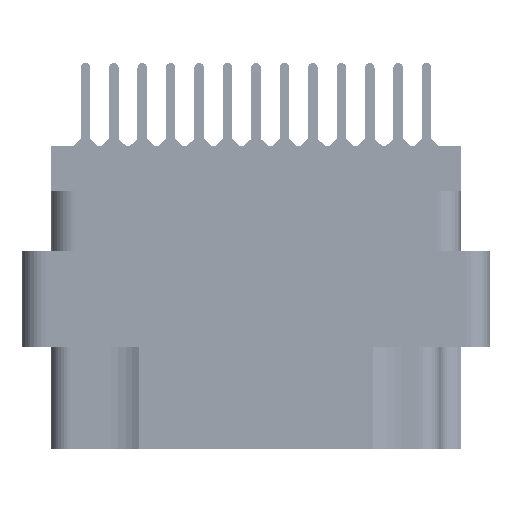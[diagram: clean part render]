
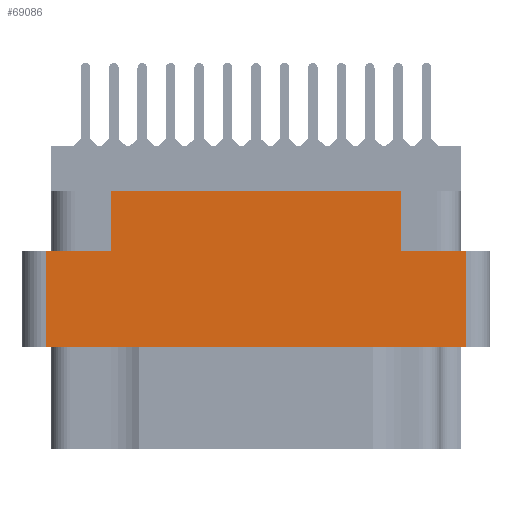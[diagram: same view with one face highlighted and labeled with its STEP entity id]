
A CAD part, left-side view. The second image highlights one B-rep face of the part: STEP entity #69086.
In plain terms, the highlighted planar face has unit normal (-1, 0, 0).
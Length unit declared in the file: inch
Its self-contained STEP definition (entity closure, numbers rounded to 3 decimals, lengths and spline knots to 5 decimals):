
#2115 = VERTEX_POINT ( 'NONE', #59527 ) ;
#8114 = ORIENTED_EDGE ( 'NONE', *, *, #72911, .F. ) ;
#8891 = ORIENTED_EDGE ( 'NONE', *, *, #37141, .T. ) ;
#9425 = VECTOR ( 'NONE', #20705, 39.37008 ) ;
#10020 = VECTOR ( 'NONE', #55788, 39.37008 ) ;
#10069 = DIRECTION ( 'NONE',  ( 0., 0., 1. ) ) ;
#10128 = CARTESIAN_POINT ( 'NONE',  ( -1.359, 0., -0.277 ) ) ;
#10649 = ORIENTED_EDGE ( 'NONE', *, *, #53684, .F. ) ;
#11189 = DIRECTION ( 'NONE',  ( -1., 0., 0. ) ) ;
#11497 = FACE_OUTER_BOUND ( 'NONE', #63966, .T. ) ;
#12118 = CARTESIAN_POINT ( 'NONE',  ( -1.359, -0.3825, -0.117 ) ) ;
#13114 = CARTESIAN_POINT ( 'NONE',  ( -1.359, 0.3825, -0.117 ) ) ;
#13892 = DIRECTION ( 'NONE',  ( 0., -1., 0. ) ) ;
#13907 = VERTEX_POINT ( 'NONE', #70611 ) ;
#17007 = EDGE_CURVE ( 'NONE', #26214, #62178, #38841, .T. ) ;
#17189 = VERTEX_POINT ( 'NONE', #28455 ) ;
#18447 = DIRECTION ( 'NONE',  ( 0., 0., 1. ) ) ;
#20012 = CARTESIAN_POINT ( 'NONE',  ( -1.359, 0.555, -0.798 ) ) ;
#20705 = DIRECTION ( 'NONE',  ( 0., 0., 1. ) ) ;
#21199 = DIRECTION ( 'NONE',  ( 0., -1., 0. ) ) ;
#21904 = CARTESIAN_POINT ( 'NONE',  ( -1.359, -0.555, -0.798 ) ) ;
#22113 = CARTESIAN_POINT ( 'NONE',  ( -1.359, 0.3825, -0.277 ) ) ;
#22502 = CARTESIAN_POINT ( 'NONE',  ( -1.359, -0.617, -0.798 ) ) ;
#25676 = CARTESIAN_POINT ( 'NONE',  ( -1.359, -0.555, -0.277 ) ) ;
#25785 = EDGE_CURVE ( 'NONE', #2115, #62178, #66826, .T. ) ;
#26214 = VERTEX_POINT ( 'NONE', #46643 ) ;
#26564 = VERTEX_POINT ( 'NONE', #67850 ) ;
#28455 = CARTESIAN_POINT ( 'NONE',  ( -1.359, 0.555, -0.277 ) ) ;
#29188 = LINE ( 'NONE', #44236, #9425 ) ;
#30741 = LINE ( 'NONE', #49799, #10020 ) ;
#30987 = CARTESIAN_POINT ( 'NONE',  ( -1.359, 0., -0.277 ) ) ;
#33061 = AXIS2_PLACEMENT_3D ( 'NONE', #22502, #11189, #18447 ) ;
#34282 = CARTESIAN_POINT ( 'NONE',  ( -1.359, 0., -0.529 ) ) ;
#34528 = DIRECTION ( 'NONE',  ( 0., 1., 0. ) ) ;
#35533 = EDGE_CURVE ( 'NONE', #17189, #13907, #43742, .T. ) ;
#37141 = EDGE_CURVE ( 'NONE', #2115, #40051, #29188, .T. ) ;
#38841 = LINE ( 'NONE', #21904, #63868 ) ;
#39416 = ORIENTED_EDGE ( 'NONE', *, *, #43409, .F. ) ;
#40051 = VERTEX_POINT ( 'NONE', #12118 ) ;
#40675 = ORIENTED_EDGE ( 'NONE', *, *, #17007, .T. ) ;
#42794 = ORIENTED_EDGE ( 'NONE', *, *, #25785, .F. ) ;
#43154 = VECTOR ( 'NONE', #60300, 39.37008 ) ;
#43409 = EDGE_CURVE ( 'NONE', #13907, #48974, #57511, .T. ) ;
#43742 = LINE ( 'NONE', #10128, #59783 ) ;
#44236 = CARTESIAN_POINT ( 'NONE',  ( -1.359, -0.3825, -0.277 ) ) ;
#44693 = ORIENTED_EDGE ( 'NONE', *, *, #35533, .F. ) ;
#46385 = LINE ( 'NONE', #34282, #54379 ) ;
#46643 = CARTESIAN_POINT ( 'NONE',  ( -1.359, -0.555, -0.529 ) ) ;
#48974 = VERTEX_POINT ( 'NONE', #13114 ) ;
#49799 = CARTESIAN_POINT ( 'NONE',  ( -1.359, 0.617, -0.117 ) ) ;
#51576 = VECTOR ( 'NONE', #13892, 39.37008 ) ;
#53684 = EDGE_CURVE ( 'NONE', #26214, #26564, #46385, .T. ) ;
#54379 = VECTOR ( 'NONE', #34528, 39.37008 ) ;
#55788 = DIRECTION ( 'NONE',  ( 0., -1., 0. ) ) ;
#56762 = PLANE ( 'NONE',  #33061 ) ;
#57511 = LINE ( 'NONE', #22113, #64702 ) ;
#57531 = EDGE_CURVE ( 'NONE', #17189, #26564, #67301, .T. ) ;
#58658 = ORIENTED_EDGE ( 'NONE', *, *, #57531, .T. ) ;
#59527 = CARTESIAN_POINT ( 'NONE',  ( -1.359, -0.3825, -0.277 ) ) ;
#59783 = VECTOR ( 'NONE', #21199, 39.37008 ) ;
#60300 = DIRECTION ( 'NONE',  ( 0., 0., -1. ) ) ;
#62178 = VERTEX_POINT ( 'NONE', #25676 ) ;
#63868 = VECTOR ( 'NONE', #68208, 39.37008 ) ;
#63966 = EDGE_LOOP ( 'NONE', ( #44693, #58658, #10649, #40675, #42794, #8891, #8114, #39416 ) ) ;
#64702 = VECTOR ( 'NONE', #10069, 39.37008 ) ;
#66826 = LINE ( 'NONE', #30987, #51576 ) ;
#67301 = LINE ( 'NONE', #20012, #43154 ) ;
#67850 = CARTESIAN_POINT ( 'NONE',  ( -1.359, 0.555, -0.529 ) ) ;
#68208 = DIRECTION ( 'NONE',  ( 0., 0., 1. ) ) ;
#69086 = ADVANCED_FACE ( 'NONE', ( #11497 ), #56762, .T. ) ;
#70611 = CARTESIAN_POINT ( 'NONE',  ( -1.359, 0.3825, -0.277 ) ) ;
#72911 = EDGE_CURVE ( 'NONE', #48974, #40051, #30741, .T. ) ;
